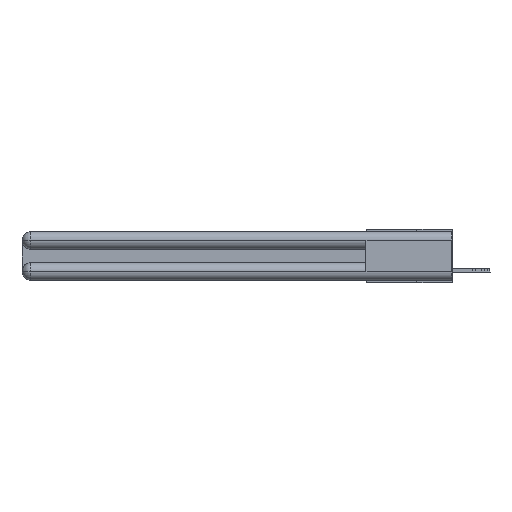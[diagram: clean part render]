
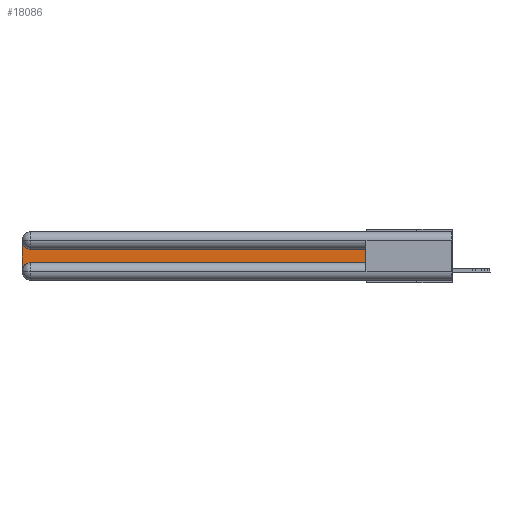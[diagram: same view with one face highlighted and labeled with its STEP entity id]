
A CAD part, left-side view. The second image highlights one B-rep face of the part: STEP entity #18086.
In plain terms, the highlighted planar face has unit normal (-1, 0, 0).
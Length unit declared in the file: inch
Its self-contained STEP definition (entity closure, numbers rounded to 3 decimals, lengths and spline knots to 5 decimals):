
#236 = VECTOR ( 'NONE', #16538, 39.37008 ) ;
#1482 = VECTOR ( 'NONE', #27665, 39.37008 ) ;
#1774 = CARTESIAN_POINT ( 'NONE',  ( 0.075, 2.94, -0.0625 ) ) ;
#2142 = ORIENTED_EDGE ( 'NONE', *, *, #18908, .T. ) ;
#3932 = VERTEX_POINT ( 'NONE', #28009 ) ;
#4279 = VERTEX_POINT ( 'NONE', #25152 ) ;
#5049 = VECTOR ( 'NONE', #5770, 39.37008 ) ;
#5282 = EDGE_CURVE ( 'NONE', #23743, #7885, #8053, .T. ) ;
#5736 = EDGE_CURVE ( 'NONE', #4279, #19689, #22991, .T. ) ;
#5770 = DIRECTION ( 'NONE',  ( 0., 1., 0. ) ) ;
#6487 = DIRECTION ( 'NONE',  ( 0., 0., -1. ) ) ;
#7885 = VERTEX_POINT ( 'NONE', #19507 ) ;
#8053 = CIRCLE ( 'NONE', #10049, 0.06 ) ;
#8088 = DIRECTION ( 'NONE',  ( 0., 0., -1. ) ) ;
#8388 = EDGE_CURVE ( 'NONE', #28477, #4279, #17650, .T. ) ;
#9583 = EDGE_CURVE ( 'NONE', #3932, #28477, #19312, .T. ) ;
#10049 = AXIS2_PLACEMENT_3D ( 'NONE', #26476, #10790, #6487 ) ;
#10790 = DIRECTION ( 'NONE',  ( 1., 0., 0. ) ) ;
#10875 = CARTESIAN_POINT ( 'NONE',  ( 0.075, 3., -0.2775 ) ) ;
#11235 = CARTESIAN_POINT ( 'NONE',  ( 0.075, 0.6, -0.2175 ) ) ;
#11546 = ORIENTED_EDGE ( 'NONE', *, *, #9583, .T. ) ;
#12068 = CARTESIAN_POINT ( 'NONE',  ( 0.075, 3., -0.2175 ) ) ;
#12510 = CARTESIAN_POINT ( 'NONE',  ( 0.075, 3., -0.1225 ) ) ;
#14491 = CARTESIAN_POINT ( 'NONE',  ( 0.075, 3., -0.0625 ) ) ;
#14597 = CARTESIAN_POINT ( 'NONE',  ( 0.075, 0.6, -0.1225 ) ) ;
#15740 = DIRECTION ( 'NONE',  ( 0., 0., 1. ) ) ;
#16538 = DIRECTION ( 'NONE',  ( 0., 0., -1. ) ) ;
#17190 = DIRECTION ( 'NONE',  ( 0., 0., -1. ) ) ;
#17206 = ORIENTED_EDGE ( 'NONE', *, *, #5736, .T. ) ;
#17650 = LINE ( 'NONE', #14597, #5049 ) ;
#18086 = ADVANCED_FACE ( 'NONE', ( #27714 ), #28163, .F. ) ;
#18908 = EDGE_CURVE ( 'NONE', #7885, #3932, #21025, .T. ) ;
#19312 = LINE ( 'NONE', #11235, #22107 ) ;
#19507 = CARTESIAN_POINT ( 'NONE',  ( 0.075, 2.94, -0.2175 ) ) ;
#19519 = DIRECTION ( 'NONE',  ( 1., 0., 0. ) ) ;
#19618 = AXIS2_PLACEMENT_3D ( 'NONE', #12510, #28069, #8088 ) ;
#19689 = VERTEX_POINT ( 'NONE', #14491 ) ;
#20835 = EDGE_CURVE ( 'NONE', #19689, #23743, #23933, .T. ) ;
#21025 = LINE ( 'NONE', #28063, #1482 ) ;
#21374 = ORIENTED_EDGE ( 'NONE', *, *, #5282, .T. ) ;
#22107 = VECTOR ( 'NONE', #15740, 39.37008 ) ;
#22238 = ORIENTED_EDGE ( 'NONE', *, *, #8388, .T. ) ;
#22991 = CIRCLE ( 'NONE', #27231, 0.06 ) ;
#23743 = VERTEX_POINT ( 'NONE', #10875 ) ;
#23933 = LINE ( 'NONE', #12068, #236 ) ;
#25152 = CARTESIAN_POINT ( 'NONE',  ( 0.075, 2.94, -0.1225 ) ) ;
#26476 = CARTESIAN_POINT ( 'NONE',  ( 0.075, 2.94, -0.2775 ) ) ;
#26650 = ORIENTED_EDGE ( 'NONE', *, *, #20835, .T. ) ;
#27231 = AXIS2_PLACEMENT_3D ( 'NONE', #1774, #19519, #17190 ) ;
#27268 = CARTESIAN_POINT ( 'NONE',  ( 0.075, 0.6, -0.1225 ) ) ;
#27665 = DIRECTION ( 'NONE',  ( 0., -1., 0. ) ) ;
#27714 = FACE_OUTER_BOUND ( 'NONE', #28852, .T. ) ;
#28009 = CARTESIAN_POINT ( 'NONE',  ( 0.075, 0.6, -0.2175 ) ) ;
#28063 = CARTESIAN_POINT ( 'NONE',  ( 0.075, 0.6, -0.2175 ) ) ;
#28069 = DIRECTION ( 'NONE',  ( 1., 0., 0. ) ) ;
#28163 = PLANE ( 'NONE',  #19618 ) ;
#28477 = VERTEX_POINT ( 'NONE', #27268 ) ;
#28852 = EDGE_LOOP ( 'NONE', ( #22238, #17206, #26650, #21374, #2142, #11546 ) ) ;
